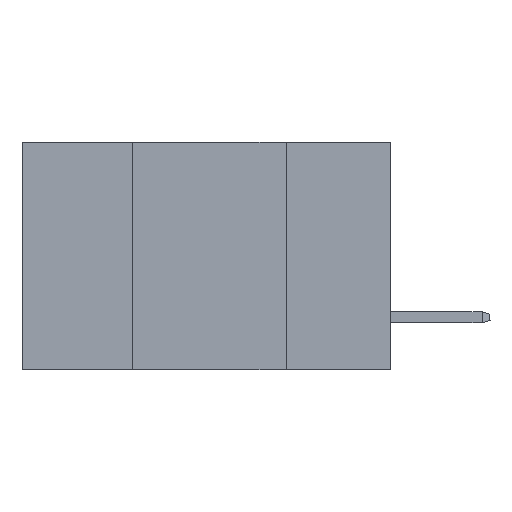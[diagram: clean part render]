
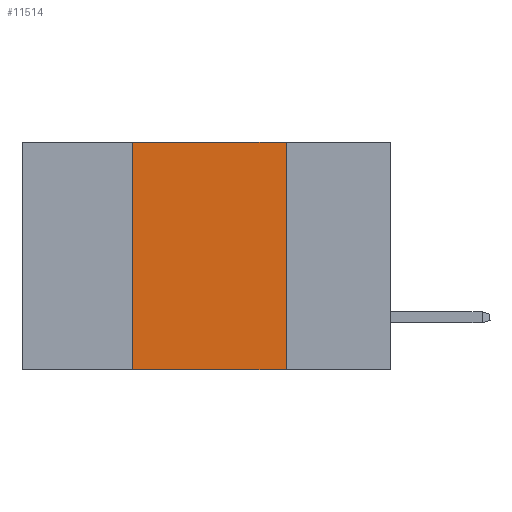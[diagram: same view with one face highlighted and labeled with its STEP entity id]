
A CAD part, left-side view. The second image highlights one B-rep face of the part: STEP entity #11514.
In plain terms, the highlighted planar face has unit normal (-1, 0, 0).
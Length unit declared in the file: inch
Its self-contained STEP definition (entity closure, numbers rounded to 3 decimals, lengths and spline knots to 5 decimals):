
#647 = LINE ( 'NONE', #20321, #16804 ) ;
#3179 = VECTOR ( 'NONE', #20178, 39.37008 ) ;
#3966 = EDGE_CURVE ( 'NONE', #5886, #13526, #6018, .T. ) ;
#5423 = DIRECTION ( 'NONE',  ( 0., 0., -1. ) ) ;
#5886 = VERTEX_POINT ( 'NONE', #11604 ) ;
#6018 = LINE ( 'NONE', #23604, #16659 ) ;
#6129 = VERTEX_POINT ( 'NONE', #10174 ) ;
#6372 = FACE_OUTER_BOUND ( 'NONE', #12140, .T. ) ;
#7735 = AXIS2_PLACEMENT_3D ( 'NONE', #12123, #16718, #5423 ) ;
#10174 = CARTESIAN_POINT ( 'NONE',  ( 0., 0.42, -0.37 ) ) ;
#11514 = ADVANCED_FACE ( 'NONE', ( #6372 ), #14833, .F. ) ;
#11604 = CARTESIAN_POINT ( 'NONE',  ( 0., 0.17, 0. ) ) ;
#12123 = CARTESIAN_POINT ( 'NONE',  ( 0., 0.6, 0. ) ) ;
#12140 = EDGE_LOOP ( 'NONE', ( #23968, #15080, #13700, #22464 ) ) ;
#13526 = VERTEX_POINT ( 'NONE', #24213 ) ;
#13700 = ORIENTED_EDGE ( 'NONE', *, *, #16728, .F. ) ;
#13936 = DIRECTION ( 'NONE',  ( 0., -1., 0. ) ) ;
#14097 = CARTESIAN_POINT ( 'NONE',  ( 0., 0.6, 0. ) ) ;
#14716 = DIRECTION ( 'NONE',  ( 0., 0., 1. ) ) ;
#14833 = PLANE ( 'NONE',  #7735 ) ;
#15080 = ORIENTED_EDGE ( 'NONE', *, *, #15994, .F. ) ;
#15994 = EDGE_CURVE ( 'NONE', #19946, #5886, #19175, .T. ) ;
#16659 = VECTOR ( 'NONE', #18205, 39.37008 ) ;
#16718 = DIRECTION ( 'NONE',  ( 1., 0., 0. ) ) ;
#16728 = EDGE_CURVE ( 'NONE', #6129, #19946, #647, .T. ) ;
#16804 = VECTOR ( 'NONE', #14716, 39.37008 ) ;
#18006 = VECTOR ( 'NONE', #13936, 39.37008 ) ;
#18205 = DIRECTION ( 'NONE',  ( 0., 0., -1. ) ) ;
#18343 = CARTESIAN_POINT ( 'NONE',  ( 0., 0.6, -0.37 ) ) ;
#19175 = LINE ( 'NONE', #14097, #18006 ) ;
#19742 = CARTESIAN_POINT ( 'NONE',  ( 0., 0.42, 0. ) ) ;
#19946 = VERTEX_POINT ( 'NONE', #19742 ) ;
#20178 = DIRECTION ( 'NONE',  ( 0., -1., 0. ) ) ;
#20272 = LINE ( 'NONE', #18343, #3179 ) ;
#20321 = CARTESIAN_POINT ( 'NONE',  ( 0., 0.42, 0. ) ) ;
#22464 = ORIENTED_EDGE ( 'NONE', *, *, #23888, .T. ) ;
#23604 = CARTESIAN_POINT ( 'NONE',  ( 0., 0.17, 0. ) ) ;
#23888 = EDGE_CURVE ( 'NONE', #6129, #13526, #20272, .T. ) ;
#23968 = ORIENTED_EDGE ( 'NONE', *, *, #3966, .F. ) ;
#24213 = CARTESIAN_POINT ( 'NONE',  ( 0., 0.17, -0.37 ) ) ;
